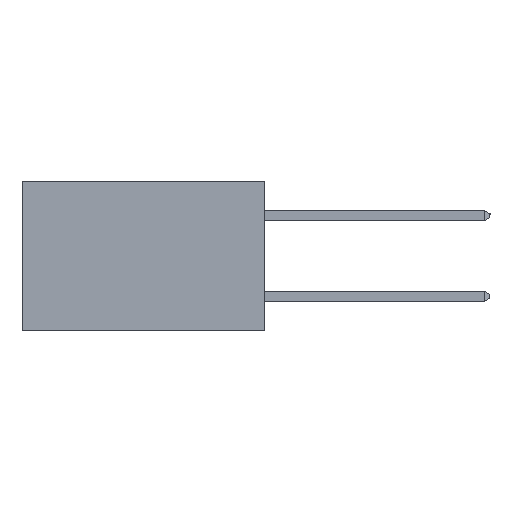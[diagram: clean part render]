
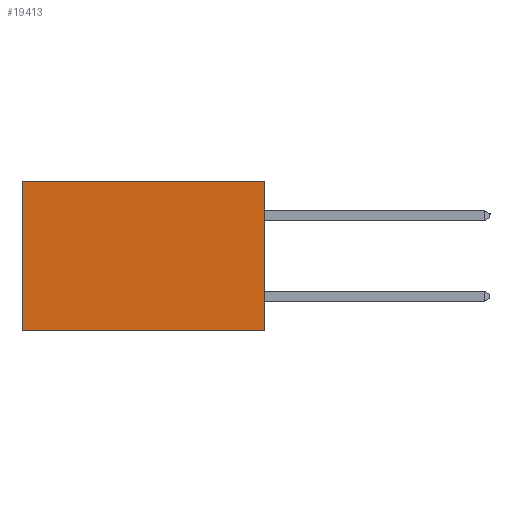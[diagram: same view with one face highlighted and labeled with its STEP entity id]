
A CAD part, left-side view. The second image highlights one B-rep face of the part: STEP entity #19413.
In plain terms, the highlighted planar face has unit normal (-1, 0, 0).
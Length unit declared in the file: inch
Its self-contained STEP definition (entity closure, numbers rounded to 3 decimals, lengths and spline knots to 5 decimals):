
#1417 = VECTOR ( 'NONE', #10681, 39.37008 ) ;
#1544 = VERTEX_POINT ( 'NONE', #22410 ) ;
#2234 = LINE ( 'NONE', #17598, #3366 ) ;
#2424 = ORIENTED_EDGE ( 'NONE', *, *, #5370, .T. ) ;
#2759 = EDGE_CURVE ( 'NONE', #4447, #1544, #2234, .T. ) ;
#3366 = VECTOR ( 'NONE', #17862, 39.37008 ) ;
#3548 = VECTOR ( 'NONE', #5385, 39.37008 ) ;
#4073 = VECTOR ( 'NONE', #7271, 39.37008 ) ;
#4268 = CARTESIAN_POINT ( 'NONE',  ( 0.298, 0.6, 0. ) ) ;
#4447 = VERTEX_POINT ( 'NONE', #11297 ) ;
#5370 = EDGE_CURVE ( 'NONE', #1544, #7247, #7833, .T. ) ;
#5385 = DIRECTION ( 'NONE',  ( 0., 0., -1. ) ) ;
#7029 = CARTESIAN_POINT ( 'NONE',  ( 0.298, 0., 0. ) ) ;
#7247 = VERTEX_POINT ( 'NONE', #21941 ) ;
#7271 = DIRECTION ( 'NONE',  ( 0., 1., 0. ) ) ;
#7348 = FACE_OUTER_BOUND ( 'NONE', #9352, .T. ) ;
#7833 = LINE ( 'NONE', #4268, #3548 ) ;
#8511 = PLANE ( 'NONE',  #14534 ) ;
#9352 = EDGE_LOOP ( 'NONE', ( #2424, #17980, #18169, #9948 ) ) ;
#9948 = ORIENTED_EDGE ( 'NONE', *, *, #2759, .T. ) ;
#10316 = DIRECTION ( 'NONE',  ( 0., 0., -1. ) ) ;
#10681 = DIRECTION ( 'NONE',  ( 0., 0., -1. ) ) ;
#11297 = CARTESIAN_POINT ( 'NONE',  ( 0.298, 0., 0. ) ) ;
#14534 = AXIS2_PLACEMENT_3D ( 'NONE', #22660, #21049, #10316 ) ;
#15315 = VERTEX_POINT ( 'NONE', #16086 ) ;
#15909 = LINE ( 'NONE', #7029, #1417 ) ;
#16054 = EDGE_CURVE ( 'NONE', #15315, #7247, #23087, .T. ) ;
#16086 = CARTESIAN_POINT ( 'NONE',  ( 0.298, 0., -0.37 ) ) ;
#16284 = CARTESIAN_POINT ( 'NONE',  ( 0.298, 0., -0.37 ) ) ;
#17598 = CARTESIAN_POINT ( 'NONE',  ( 0.298, 0., 0. ) ) ;
#17862 = DIRECTION ( 'NONE',  ( 0., 1., 0. ) ) ;
#17980 = ORIENTED_EDGE ( 'NONE', *, *, #16054, .F. ) ;
#18169 = ORIENTED_EDGE ( 'NONE', *, *, #18342, .F. ) ;
#18342 = EDGE_CURVE ( 'NONE', #4447, #15315, #15909, .T. ) ;
#19413 = ADVANCED_FACE ( 'NONE', ( #7348 ), #8511, .F. ) ;
#21049 = DIRECTION ( 'NONE',  ( 1., 0., 0. ) ) ;
#21941 = CARTESIAN_POINT ( 'NONE',  ( 0.298, 0.6, -0.37 ) ) ;
#22410 = CARTESIAN_POINT ( 'NONE',  ( 0.298, 0.6, 0. ) ) ;
#22660 = CARTESIAN_POINT ( 'NONE',  ( 0.298, 0., 0. ) ) ;
#23087 = LINE ( 'NONE', #16284, #4073 ) ;
